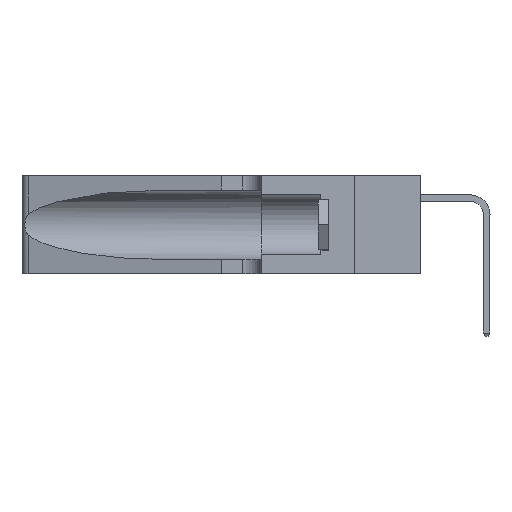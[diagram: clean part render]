
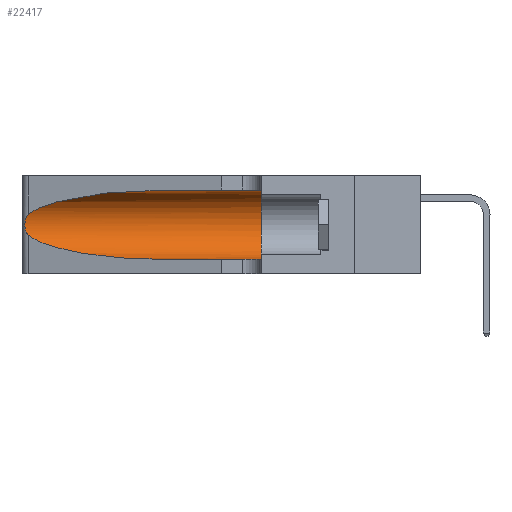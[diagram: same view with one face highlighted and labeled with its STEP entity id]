
A CAD part, left-side view. The second image highlights one B-rep face of the part: STEP entity #22417.
In plain terms, the highlighted cylindrical face has radius 3.308 mm (diameter 6.617 mm), a partial arc.
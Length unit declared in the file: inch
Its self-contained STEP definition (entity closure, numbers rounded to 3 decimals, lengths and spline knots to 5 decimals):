
#820 = EDGE_CURVE ( 'NONE', #8187, #19848, #16301, .T. ) ;
#934 = AXIS2_PLACEMENT_3D ( 'NONE', #14430, #19012, #9797 ) ;
#1028 = CARTESIAN_POINT ( 'NONE',  ( 0.25789, 1.23486, 0.15765 ) ) ;
#1158 = B_SPLINE_CURVE_WITH_KNOTS ( 'NONE', 3,
 ( #17314, #24163, #21924, #8112, #24262, #10516, #26548, #12819, #28852, #15122, #1028, #17421, #3468, #19700 ),
 .UNSPECIFIED., .F., .F.,
 ( 4, 2, 2, 2, 2, 2, 4 ),
 ( 0., 0.00027, 0.00053, 0.00107, 0.0016, 0.00187, 0.00214 ),
 .UNSPECIFIED. ) ;
#2044 = ORIENTED_EDGE ( 'NONE', *, *, #820, .F. ) ;
#2168 = CARTESIAN_POINT ( 'NONE',  ( 0.1305, 0.72297, 0.31525 ) ) ;
#2860 = EDGE_CURVE ( 'NONE', #25147, #8187, #9395, .T. ) ;
#2901 =( BOUNDED_CURVE ( )  B_SPLINE_CURVE ( 3, ( #2168, #4564, #13895, #6905 ),
 .UNSPECIFIED., .F., .F. ) 
 B_SPLINE_CURVE_WITH_KNOTS ( ( 4, 4 ),
 ( 1.5708, 2.84003 ),
 .UNSPECIFIED. ) 
 CURVE ( )  GEOMETRIC_REPRESENTATION_ITEM ( )  RATIONAL_B_SPLINE_CURVE ( ( 1., 0.87, 0.87, 1. ) ) 
 REPRESENTATION_ITEM ( '' )  );
#3468 = CARTESIAN_POINT ( 'NONE',  ( 0.25555, 1.22993, 0.14849 ) ) ;
#3609 = DIRECTION ( 'NONE',  ( 0., -1., 0. ) ) ;
#4564 = CARTESIAN_POINT ( 'NONE',  ( 0.18966, 0.96281, 0.31525 ) ) ;
#5481 = DIRECTION ( 'NONE',  ( 0., -1., 0. ) ) ;
#5771 = CARTESIAN_POINT ( 'NONE',  ( 0.1305, 0.72297, 0.31525 ) ) ;
#6887 =( BOUNDED_CURVE ( )  B_SPLINE_CURVE ( 3, ( #20726, #11539, #29984, #16227 ),
 .UNSPECIFIED., .F., .F. ) 
 B_SPLINE_CURVE_WITH_KNOTS ( ( 4, 4 ),
 ( 3.44316, 4.71239 ),
 .UNSPECIFIED. ) 
 CURVE ( )  GEOMETRIC_REPRESENTATION_ITEM ( )  RATIONAL_B_SPLINE_CURVE ( ( 1., 0.87, 0.87, 1. ) ) 
 REPRESENTATION_ITEM ( '' )  );
#6905 = CARTESIAN_POINT ( 'NONE',  ( 0.25487, 1.22718, 0.22369 ) ) ;
#7660 = DIRECTION ( 'NONE',  ( 0., 0., 1. ) ) ;
#7697 = CARTESIAN_POINT ( 'NONE',  ( 0.1305, 0.35, 0.185 ) ) ;
#8112 = CARTESIAN_POINT ( 'NONE',  ( 0.25787, 1.23484, 0.2124 ) ) ;
#8187 = VERTEX_POINT ( 'NONE', #26884 ) ;
#8281 = VERTEX_POINT ( 'NONE', #20342 ) ;
#8373 = CARTESIAN_POINT ( 'NONE',  ( 0.1305, 1.61858, 0.05475 ) ) ;
#8544 = VECTOR ( 'NONE', #3609, 39.37008 ) ;
#8644 = VECTOR ( 'NONE', #5481, 39.37008 ) ;
#9395 = LINE ( 'NONE', #12579, #8644 ) ;
#9797 = DIRECTION ( 'NONE',  ( 0., 0., -1. ) ) ;
#10516 = CARTESIAN_POINT ( 'NONE',  ( 0.26018, 1.23835, 0.19895 ) ) ;
#10988 = EDGE_LOOP ( 'NONE', ( #15123, #25764, #24026, #25026, #2044, #23478 ) ) ;
#11539 = CARTESIAN_POINT ( 'NONE',  ( 0.2373, 1.15595, 0.08982 ) ) ;
#11690 = VERTEX_POINT ( 'NONE', #25345 ) ;
#12579 = CARTESIAN_POINT ( 'NONE',  ( 0.1305, 1.61858, 0.31525 ) ) ;
#12819 = CARTESIAN_POINT ( 'NONE',  ( 0.26075, 1.23896, 0.178 ) ) ;
#13895 = CARTESIAN_POINT ( 'NONE',  ( 0.2373, 1.15595, 0.28018 ) ) ;
#14430 = CARTESIAN_POINT ( 'NONE',  ( 0.1305, 1.61858, 0.185 ) ) ;
#15122 = CARTESIAN_POINT ( 'NONE',  ( 0.25856, 1.23593, 0.16098 ) ) ;
#15123 = ORIENTED_EDGE ( 'NONE', *, *, #17834, .T. ) ;
#15746 = CYLINDRICAL_SURFACE ( 'NONE', #934, 0.13025 ) ;
#16227 = CARTESIAN_POINT ( 'NONE',  ( 0.1305, 0.72297, 0.05475 ) ) ;
#16301 = CIRCLE ( 'NONE', #28426, 0.13025 ) ;
#16329 = EDGE_CURVE ( 'NONE', #8281, #19848, #20780, .T. ) ;
#17314 = CARTESIAN_POINT ( 'NONE',  ( 0.25487, 1.22718, 0.22369 ) ) ;
#17421 = CARTESIAN_POINT ( 'NONE',  ( 0.25639, 1.23186, 0.15144 ) ) ;
#17834 = EDGE_CURVE ( 'NONE', #25147, #19166, #2901, .T. ) ;
#18781 = EDGE_CURVE ( 'NONE', #19166, #11690, #1158, .T. ) ;
#19012 = DIRECTION ( 'NONE',  ( 0., -1., 0. ) ) ;
#19166 = VERTEX_POINT ( 'NONE', #22676 ) ;
#19700 = CARTESIAN_POINT ( 'NONE',  ( 0.25487, 1.22718, 0.14631 ) ) ;
#19848 = VERTEX_POINT ( 'NONE', #23341 ) ;
#20342 = CARTESIAN_POINT ( 'NONE',  ( 0.1305, 0.72297, 0.05475 ) ) ;
#20726 = CARTESIAN_POINT ( 'NONE',  ( 0.25487, 1.22718, 0.14631 ) ) ;
#20780 = LINE ( 'NONE', #8373, #8544 ) ;
#21924 = CARTESIAN_POINT ( 'NONE',  ( 0.25639, 1.23184, 0.21858 ) ) ;
#22417 = ADVANCED_FACE ( 'NONE', ( #22566 ), #15746, .F. ) ;
#22566 = FACE_OUTER_BOUND ( 'NONE', #10988, .T. ) ;
#22676 = CARTESIAN_POINT ( 'NONE',  ( 0.25487, 1.22718, 0.22369 ) ) ;
#23341 = CARTESIAN_POINT ( 'NONE',  ( 0.1305, 0.35, 0.05475 ) ) ;
#23478 = ORIENTED_EDGE ( 'NONE', *, *, #2860, .F. ) ;
#24026 = ORIENTED_EDGE ( 'NONE', *, *, #28722, .T. ) ;
#24163 = CARTESIAN_POINT ( 'NONE',  ( 0.25555, 1.22994, 0.2215 ) ) ;
#24262 = CARTESIAN_POINT ( 'NONE',  ( 0.25854, 1.2359, 0.20912 ) ) ;
#25026 = ORIENTED_EDGE ( 'NONE', *, *, #16329, .T. ) ;
#25147 = VERTEX_POINT ( 'NONE', #5771 ) ;
#25345 = CARTESIAN_POINT ( 'NONE',  ( 0.25487, 1.22718, 0.14631 ) ) ;
#25764 = ORIENTED_EDGE ( 'NONE', *, *, #18781, .T. ) ;
#26548 = CARTESIAN_POINT ( 'NONE',  ( 0.26075, 1.23896, 0.19203 ) ) ;
#26884 = CARTESIAN_POINT ( 'NONE',  ( 0.1305, 0.35, 0.31525 ) ) ;
#28426 = AXIS2_PLACEMENT_3D ( 'NONE', #7697, #28738, #7660 ) ;
#28722 = EDGE_CURVE ( 'NONE', #11690, #8281, #6887, .T. ) ;
#28738 = DIRECTION ( 'NONE',  ( 0., 1., 0. ) ) ;
#28852 = CARTESIAN_POINT ( 'NONE',  ( 0.26017, 1.23833, 0.17102 ) ) ;
#29984 = CARTESIAN_POINT ( 'NONE',  ( 0.18966, 0.96281, 0.05475 ) ) ;
